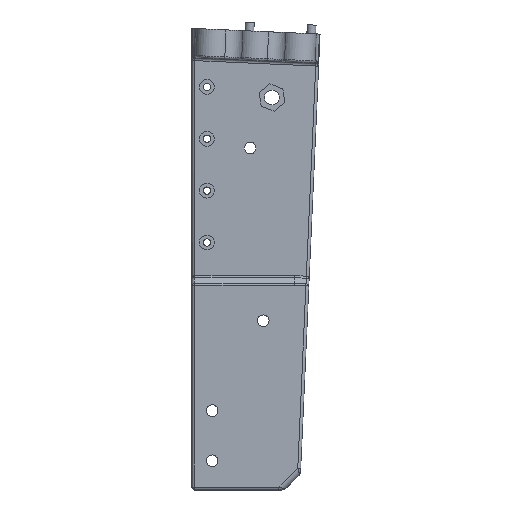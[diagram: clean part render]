
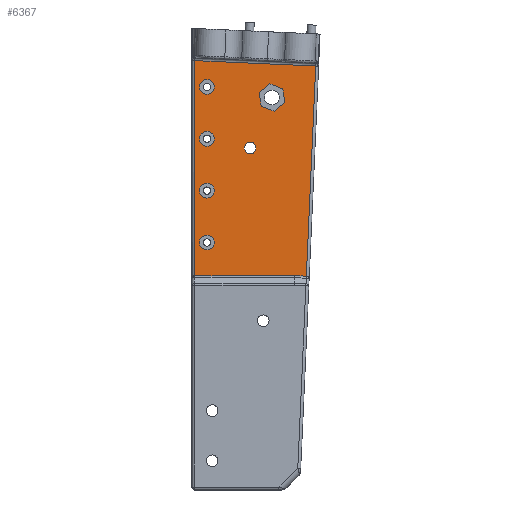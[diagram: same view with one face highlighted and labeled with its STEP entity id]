
A CAD part, left-side view. The second image highlights one B-rep face of the part: STEP entity #6367.
In plain terms, the highlighted planar face has unit normal (-1, 0, 0).
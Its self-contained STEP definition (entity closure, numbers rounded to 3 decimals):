
#206=FACE_BOUND('',#1096,.T.);
#207=FACE_BOUND('',#1097,.T.);
#208=FACE_BOUND('',#1098,.T.);
#209=FACE_BOUND('',#1099,.T.);
#210=FACE_BOUND('',#1100,.T.);
#211=FACE_BOUND('',#1101,.T.);
#329=PLANE('',#6980);
#444=ELLIPSE('',#6926,2.83,2.);
#680=FACE_OUTER_BOUND('',#1095,.T.);
#1095=EDGE_LOOP('',(#5348,#5349,#5350,#5351,#5352,#5353));
#1096=EDGE_LOOP('',(#5354,#5355,#5356,#5357,#5358,#5359));
#1097=EDGE_LOOP('',(#5360,#5361));
#1098=EDGE_LOOP('',(#5362,#5363));
#1099=EDGE_LOOP('',(#5364,#5365));
#1100=EDGE_LOOP('',(#5366,#5367));
#1101=EDGE_LOOP('',(#5368,#5369));
#1563=LINE('',#10080,#2109);
#1567=LINE('',#10088,#2113);
#1570=LINE('',#10094,#2116);
#1573=LINE('',#10100,#2119);
#1576=LINE('',#10106,#2122);
#1579=LINE('',#10111,#2125);
#1617=LINE('',#10739,#2163);
#1636=LINE('',#11366,#2182);
#1638=LINE('',#11393,#2184);
#1646=LINE('',#11434,#2192);
#1647=LINE('',#11436,#2193);
#2109=VECTOR('',#7798,10.);
#2113=VECTOR('',#7804,10.);
#2116=VECTOR('',#7809,10.);
#2119=VECTOR('',#7814,10.);
#2122=VECTOR('',#7819,10.);
#2125=VECTOR('',#7824,10.);
#2163=VECTOR('',#8146,10.);
#2182=VECTOR('',#8341,10.);
#2184=VECTOR('',#8353,10.);
#2192=VECTOR('',#8379,10.);
#2193=VECTOR('',#8382,10.);
#2417=CIRCLE('',#6714,2.54);
#2418=CIRCLE('',#6715,2.54);
#2422=CIRCLE('',#6721,2.54);
#2423=CIRCLE('',#6722,2.54);
#2427=CIRCLE('',#6728,2.54);
#2428=CIRCLE('',#6729,2.54);
#2432=CIRCLE('',#6735,2.54);
#2433=CIRCLE('',#6736,2.54);
#2572=CIRCLE('',#6981,2.);
#2573=CIRCLE('',#6982,2.);
#2938=VERTEX_POINT('',#10078);
#2939=VERTEX_POINT('',#10079);
#2942=VERTEX_POINT('',#10087);
#2944=VERTEX_POINT('',#10093);
#2946=VERTEX_POINT('',#10099);
#2948=VERTEX_POINT('',#10105);
#2961=VERTEX_POINT('',#10155);
#2962=VERTEX_POINT('',#10157);
#2966=VERTEX_POINT('',#10168);
#2967=VERTEX_POINT('',#10170);
#2971=VERTEX_POINT('',#10181);
#2972=VERTEX_POINT('',#10183);
#2976=VERTEX_POINT('',#10194);
#2977=VERTEX_POINT('',#10196);
#3037=VERTEX_POINT('',#10725);
#3041=VERTEX_POINT('',#10737);
#3113=VERTEX_POINT('',#11358);
#3115=VERTEX_POINT('',#11364);
#3117=VERTEX_POINT('',#11385);
#3119=VERTEX_POINT('',#11391);
#3135=VERTEX_POINT('',#11584);
#3136=VERTEX_POINT('',#11585);
#3623=EDGE_CURVE('',#2938,#2939,#1563,.T.);
#3627=EDGE_CURVE('',#2942,#2938,#1567,.T.);
#3630=EDGE_CURVE('',#2944,#2942,#1570,.T.);
#3633=EDGE_CURVE('',#2946,#2944,#1573,.T.);
#3636=EDGE_CURVE('',#2948,#2946,#1576,.T.);
#3639=EDGE_CURVE('',#2939,#2948,#1579,.T.);
#3662=EDGE_CURVE('',#2962,#2961,#2417,.T.);
#3663=EDGE_CURVE('',#2961,#2962,#2418,.T.);
#3668=EDGE_CURVE('',#2967,#2966,#2422,.T.);
#3669=EDGE_CURVE('',#2966,#2967,#2423,.T.);
#3674=EDGE_CURVE('',#2972,#2971,#2427,.T.);
#3675=EDGE_CURVE('',#2971,#2972,#2428,.T.);
#3680=EDGE_CURVE('',#2977,#2976,#2432,.T.);
#3681=EDGE_CURVE('',#2976,#2977,#2433,.T.);
#3781=EDGE_CURVE('',#3041,#3037,#1617,.T.);
#3887=EDGE_CURVE('',#3115,#3113,#1636,.T.);
#3890=EDGE_CURVE('',#3117,#3115,#444,.T.);
#3893=EDGE_CURVE('',#3119,#3117,#1638,.T.);
#3905=EDGE_CURVE('',#3113,#3041,#1646,.T.);
#3906=EDGE_CURVE('',#3037,#3119,#1647,.T.);
#3948=EDGE_CURVE('',#3135,#3136,#2572,.T.);
#3949=EDGE_CURVE('',#3136,#3135,#2573,.T.);
#5348=ORIENTED_EDGE('',*,*,#3781,.F.);
#5349=ORIENTED_EDGE('',*,*,#3905,.F.);
#5350=ORIENTED_EDGE('',*,*,#3887,.F.);
#5351=ORIENTED_EDGE('',*,*,#3890,.F.);
#5352=ORIENTED_EDGE('',*,*,#3893,.F.);
#5353=ORIENTED_EDGE('',*,*,#3906,.F.);
#5354=ORIENTED_EDGE('',*,*,#3623,.T.);
#5355=ORIENTED_EDGE('',*,*,#3639,.T.);
#5356=ORIENTED_EDGE('',*,*,#3636,.T.);
#5357=ORIENTED_EDGE('',*,*,#3633,.T.);
#5358=ORIENTED_EDGE('',*,*,#3630,.T.);
#5359=ORIENTED_EDGE('',*,*,#3627,.T.);
#5360=ORIENTED_EDGE('',*,*,#3662,.T.);
#5361=ORIENTED_EDGE('',*,*,#3663,.T.);
#5362=ORIENTED_EDGE('',*,*,#3668,.T.);
#5363=ORIENTED_EDGE('',*,*,#3669,.T.);
#5364=ORIENTED_EDGE('',*,*,#3674,.T.);
#5365=ORIENTED_EDGE('',*,*,#3675,.T.);
#5366=ORIENTED_EDGE('',*,*,#3680,.T.);
#5367=ORIENTED_EDGE('',*,*,#3681,.T.);
#5368=ORIENTED_EDGE('',*,*,#3948,.T.);
#5369=ORIENTED_EDGE('',*,*,#3949,.T.);
#6367=ADVANCED_FACE('',(#680,#206,#207,#208,#209,#210,#211),#329,.F.);
#6714=AXIS2_PLACEMENT_3D('',#10158,#7877,#7878);
#6715=AXIS2_PLACEMENT_3D('',#10159,#7879,#7880);
#6721=AXIS2_PLACEMENT_3D('',#10171,#7892,#7893);
#6722=AXIS2_PLACEMENT_3D('',#10172,#7894,#7895);
#6728=AXIS2_PLACEMENT_3D('',#10184,#7907,#7908);
#6729=AXIS2_PLACEMENT_3D('',#10185,#7909,#7910);
#6735=AXIS2_PLACEMENT_3D('',#10197,#7922,#7923);
#6736=AXIS2_PLACEMENT_3D('',#10198,#7924,#7925);
#6926=AXIS2_PLACEMENT_3D('',#11387,#8345,#8346);
#6980=AXIS2_PLACEMENT_3D('',#11583,#8493,#8494);
#6981=AXIS2_PLACEMENT_3D('',#11586,#8495,#8496);
#6982=AXIS2_PLACEMENT_3D('',#11587,#8497,#8498);
#7798=DIRECTION('',(0.,0.153,0.988));
#7804=DIRECTION('',(0.,0.932,0.362));
#7809=DIRECTION('',(0.,0.78,-0.626));
#7814=DIRECTION('',(0.,-0.153,-0.988));
#7819=DIRECTION('',(0.,-0.932,-0.362));
#7824=DIRECTION('',(0.,-0.78,0.626));
#7877=DIRECTION('center_axis',(1.,0.,0.));
#7878=DIRECTION('ref_axis',(0.,0.,-1.));
#7879=DIRECTION('center_axis',(1.,0.,0.));
#7880=DIRECTION('ref_axis',(0.,0.,-1.));
#7892=DIRECTION('center_axis',(1.,0.,0.));
#7893=DIRECTION('ref_axis',(0.,0.,-1.));
#7894=DIRECTION('center_axis',(1.,0.,0.));
#7895=DIRECTION('ref_axis',(0.,0.,-1.));
#7907=DIRECTION('center_axis',(1.,0.,0.));
#7908=DIRECTION('ref_axis',(0.,0.,-1.));
#7909=DIRECTION('center_axis',(1.,0.,0.));
#7910=DIRECTION('ref_axis',(0.,0.,-1.));
#7922=DIRECTION('center_axis',(1.,0.,0.));
#7923=DIRECTION('ref_axis',(0.,0.,-1.));
#7924=DIRECTION('center_axis',(1.,0.,0.));
#7925=DIRECTION('ref_axis',(0.,0.,-1.));
#8146=DIRECTION('',(0.,-0.999,-0.044));
#8341=DIRECTION('',(0.,1.,0.));
#8345=DIRECTION('center_axis',(-1.,0.,0.));
#8346=DIRECTION('ref_axis',(0.,-0.044,0.999));
#8353=DIRECTION('',(0.,0.999,0.044));
#8379=DIRECTION('',(0.,0.,1.));
#8382=DIRECTION('',(0.,0.044,-0.999));
#8493=DIRECTION('center_axis',(1.,0.,0.));
#8494=DIRECTION('ref_axis',(0.,0.,-1.));
#8495=DIRECTION('center_axis',(1.,0.,0.));
#8496=DIRECTION('ref_axis',(0.,0.,1.));
#8497=DIRECTION('center_axis',(1.,0.,0.));
#8498=DIRECTION('ref_axis',(0.,0.,1.));
#10078=CARTESIAN_POINT('',(-27.1,-23.81,131.535));
#10079=CARTESIAN_POINT('',(-27.1,-23.087,136.213));
#10080=CARTESIAN_POINT('',(-27.1,-25.29,121.957));
#10087=CARTESIAN_POINT('',(-27.1,-28.223,129.821));
#10088=CARTESIAN_POINT('',(-27.1,-28.595,129.677));
#10093=CARTESIAN_POINT('',(-27.1,-31.913,132.787));
#10094=CARTESIAN_POINT('',(-27.1,-23.748,126.225));
#10099=CARTESIAN_POINT('',(-27.1,-31.19,137.465));
#10100=CARTESIAN_POINT('',(-27.1,-33.032,125.548));
#10105=CARTESIAN_POINT('',(-27.1,-26.777,139.179));
#10106=CARTESIAN_POINT('',(-27.1,-29.356,138.178));
#10111=CARTESIAN_POINT('',(-27.1,-16.766,131.134));
#10155=CARTESIAN_POINT('',(-27.1,-5.186,105.126));
#10157=CARTESIAN_POINT('',(-27.1,-5.186,100.046));
#10158=CARTESIAN_POINT('Origin',(-27.1,-5.186,102.586));
#10159=CARTESIAN_POINT('Origin',(-27.1,-5.186,102.586));
#10168=CARTESIAN_POINT('',(-27.1,-5.186,122.906));
#10170=CARTESIAN_POINT('',(-27.1,-5.186,117.826));
#10171=CARTESIAN_POINT('Origin',(-27.1,-5.186,120.366));
#10172=CARTESIAN_POINT('Origin',(-27.1,-5.186,120.366));
#10181=CARTESIAN_POINT('',(-27.1,-5.186,87.346));
#10183=CARTESIAN_POINT('',(-27.1,-5.186,82.266));
#10184=CARTESIAN_POINT('Origin',(-27.1,-5.186,84.806));
#10185=CARTESIAN_POINT('Origin',(-27.1,-5.186,84.806));
#10194=CARTESIAN_POINT('',(-27.1,-5.186,140.686));
#10196=CARTESIAN_POINT('',(-27.1,-5.186,135.606));
#10197=CARTESIAN_POINT('Origin',(-27.1,-5.186,138.146));
#10198=CARTESIAN_POINT('Origin',(-27.1,-5.186,138.146));
#10725=CARTESIAN_POINT('',(-27.1,-42.475,145.293));
#10737=CARTESIAN_POINT('',(-27.1,-1.086,147.136));
#10739=CARTESIAN_POINT('',(-27.1,-22.548,146.181));
#11358=CARTESIAN_POINT('',(-27.1,-1.086,73.456));
#11364=CARTESIAN_POINT('',(-27.1,-35.224,73.456));
#11366=CARTESIAN_POINT('',(-27.1,-11.034,73.456));
#11385=CARTESIAN_POINT('',(-27.1,-35.287,73.454));
#11387=CARTESIAN_POINT('Origin',(-27.1,-35.161,70.627));
#11391=CARTESIAN_POINT('',(-27.1,-39.267,73.277));
#11393=CARTESIAN_POINT('',(-27.1,-27.812,73.787));
#11434=CARTESIAN_POINT('',(-27.1,-1.086,55.823));
#11436=CARTESIAN_POINT('',(-27.1,-39.739,83.86));
#11583=CARTESIAN_POINT('Origin',(-27.1,-22.024,111.646));
#11584=CARTESIAN_POINT('',(-27.1,-20.,115.2));
#11585=CARTESIAN_POINT('',(-27.1,-20.,119.2));
#11586=CARTESIAN_POINT('Origin',(-27.1,-20.,117.2));
#11587=CARTESIAN_POINT('Origin',(-27.1,-20.,117.2));
